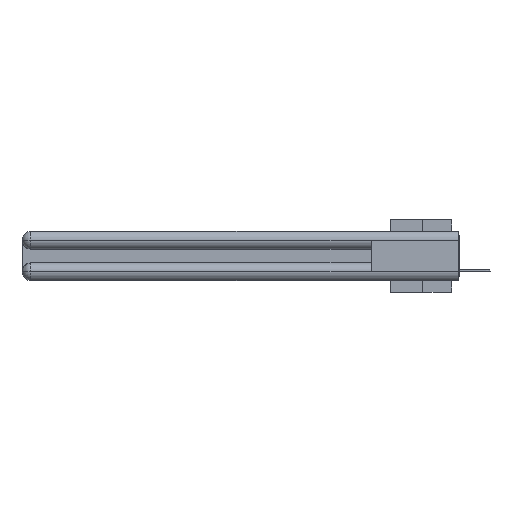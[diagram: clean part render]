
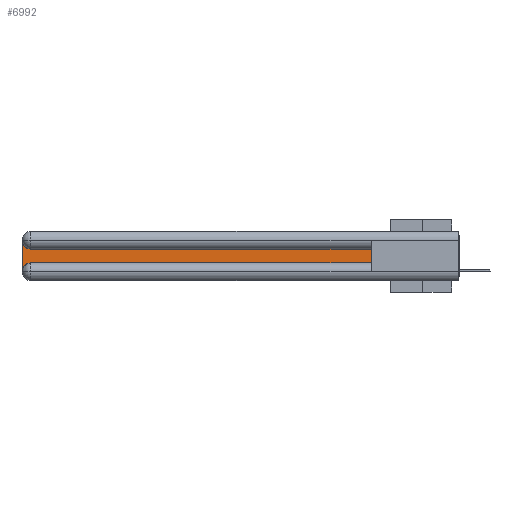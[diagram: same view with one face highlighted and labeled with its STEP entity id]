
A CAD part, left-side view. The second image highlights one B-rep face of the part: STEP entity #6992.
In plain terms, the highlighted planar face has unit normal (-1, 0, 0).
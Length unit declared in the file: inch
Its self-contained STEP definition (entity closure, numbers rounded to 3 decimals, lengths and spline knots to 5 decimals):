
#375 = CARTESIAN_POINT ( 'NONE',  ( 0.075, 2.94, -0.1225 ) ) ;
#1030 = DIRECTION ( 'NONE',  ( 0., 0., -1. ) ) ;
#1288 = DIRECTION ( 'NONE',  ( 1., 0., 0. ) ) ;
#1541 = AXIS2_PLACEMENT_3D ( 'NONE', #4571, #16546, #13212 ) ;
#3240 = EDGE_CURVE ( 'NONE', #22695, #25361, #19440, .T. ) ;
#4571 = CARTESIAN_POINT ( 'NONE',  ( 0.075, 2.94, -0.0625 ) ) ;
#6063 = VERTEX_POINT ( 'NONE', #12256 ) ;
#6992 = ADVANCED_FACE ( 'NONE', ( #11776 ), #27174, .F. ) ;
#7097 = VECTOR ( 'NONE', #24452, 39.37008 ) ;
#7773 = CARTESIAN_POINT ( 'NONE',  ( 0.075, 0.6, -0.1225 ) ) ;
#8012 = CARTESIAN_POINT ( 'NONE',  ( 0.075, 0.6, -0.1225 ) ) ;
#8780 = CARTESIAN_POINT ( 'NONE',  ( 0.075, 3., -0.2175 ) ) ;
#8951 = DIRECTION ( 'NONE',  ( 1., 0., 0. ) ) ;
#9147 = EDGE_CURVE ( 'NONE', #10583, #6063, #22525, .T. ) ;
#9462 = ORIENTED_EDGE ( 'NONE', *, *, #9147, .T. ) ;
#9821 = AXIS2_PLACEMENT_3D ( 'NONE', #31368, #1288, #1030 ) ;
#10583 = VERTEX_POINT ( 'NONE', #39052 ) ;
#10996 = EDGE_CURVE ( 'NONE', #25361, #23926, #35273, .T. ) ;
#11372 = VECTOR ( 'NONE', #30499, 39.37008 ) ;
#11775 = CARTESIAN_POINT ( 'NONE',  ( 0.075, 3., -0.1225 ) ) ;
#11776 = FACE_OUTER_BOUND ( 'NONE', #24250, .T. ) ;
#12256 = CARTESIAN_POINT ( 'NONE',  ( 0.075, 2.94, -0.2175 ) ) ;
#12474 = CARTESIAN_POINT ( 'NONE',  ( 0.075, 0.6, -0.2175 ) ) ;
#12530 = ORIENTED_EDGE ( 'NONE', *, *, #3240, .T. ) ;
#13092 = AXIS2_PLACEMENT_3D ( 'NONE', #11775, #8951, #39288 ) ;
#13212 = DIRECTION ( 'NONE',  ( 0., 0., -1. ) ) ;
#14250 = LINE ( 'NONE', #12474, #7097 ) ;
#16546 = DIRECTION ( 'NONE',  ( 1., 0., 0. ) ) ;
#17709 = DIRECTION ( 'NONE',  ( 0., 0., -1. ) ) ;
#18961 = EDGE_CURVE ( 'NONE', #6063, #22695, #14250, .T. ) ;
#19440 = LINE ( 'NONE', #36340, #11372 ) ;
#20270 = CARTESIAN_POINT ( 'NONE',  ( 0.075, 3., -0.0625 ) ) ;
#21793 = ORIENTED_EDGE ( 'NONE', *, *, #28574, .T. ) ;
#22525 = CIRCLE ( 'NONE', #9821, 0.06 ) ;
#22695 = VERTEX_POINT ( 'NONE', #31720 ) ;
#23926 = VERTEX_POINT ( 'NONE', #375 ) ;
#24250 = EDGE_LOOP ( 'NONE', ( #37714, #21793, #34015, #9462, #35204, #12530 ) ) ;
#24287 = VECTOR ( 'NONE', #17709, 39.37008 ) ;
#24452 = DIRECTION ( 'NONE',  ( 0., -1., 0. ) ) ;
#25361 = VERTEX_POINT ( 'NONE', #8012 ) ;
#25544 = EDGE_CURVE ( 'NONE', #27632, #10583, #29032, .T. ) ;
#27174 = PLANE ( 'NONE',  #13092 ) ;
#27632 = VERTEX_POINT ( 'NONE', #20270 ) ;
#28574 = EDGE_CURVE ( 'NONE', #23926, #27632, #30737, .T. ) ;
#29032 = LINE ( 'NONE', #8780, #24287 ) ;
#30499 = DIRECTION ( 'NONE',  ( 0., 0., 1. ) ) ;
#30737 = CIRCLE ( 'NONE', #1541, 0.06 ) ;
#31368 = CARTESIAN_POINT ( 'NONE',  ( 0.075, 2.94, -0.2775 ) ) ;
#31720 = CARTESIAN_POINT ( 'NONE',  ( 0.075, 0.6, -0.2175 ) ) ;
#34015 = ORIENTED_EDGE ( 'NONE', *, *, #25544, .T. ) ;
#35204 = ORIENTED_EDGE ( 'NONE', *, *, #18961, .T. ) ;
#35273 = LINE ( 'NONE', #7773, #39117 ) ;
#36340 = CARTESIAN_POINT ( 'NONE',  ( 0.075, 0.6, -0.2175 ) ) ;
#37714 = ORIENTED_EDGE ( 'NONE', *, *, #10996, .T. ) ;
#37945 = DIRECTION ( 'NONE',  ( 0., 1., 0. ) ) ;
#39052 = CARTESIAN_POINT ( 'NONE',  ( 0.075, 3., -0.2775 ) ) ;
#39117 = VECTOR ( 'NONE', #37945, 39.37008 ) ;
#39288 = DIRECTION ( 'NONE',  ( 0., 0., -1. ) ) ;
